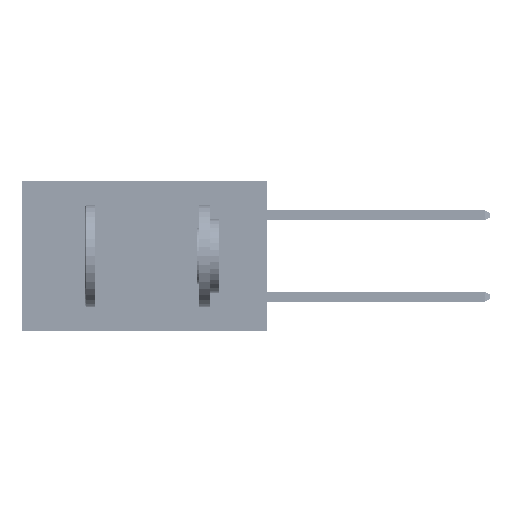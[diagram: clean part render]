
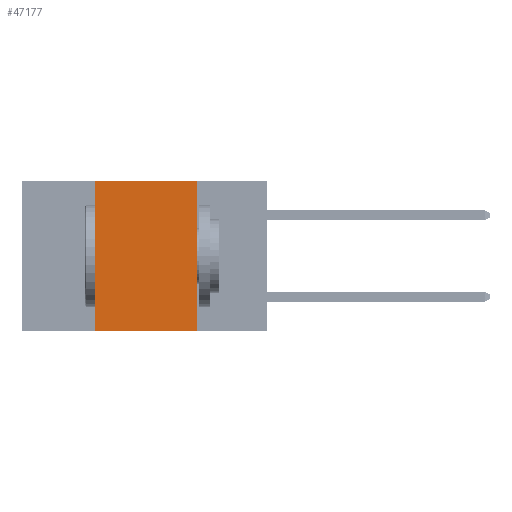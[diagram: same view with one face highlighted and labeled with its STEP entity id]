
A CAD part, left-side view. The second image highlights one B-rep face of the part: STEP entity #47177.
In plain terms, the highlighted planar face has unit normal (-1, 0, 0).
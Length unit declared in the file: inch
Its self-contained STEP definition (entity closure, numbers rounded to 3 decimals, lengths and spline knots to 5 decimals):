
#1394 = CARTESIAN_POINT ( 'NONE',  ( 0., 0.6, 0. ) ) ;
#2716 = DIRECTION ( 'NONE',  ( 0., -1., 0. ) ) ;
#3013 = EDGE_CURVE ( 'NONE', #48304, #9676, #44923, .T. ) ;
#9676 = VERTEX_POINT ( 'NONE', #44063 ) ;
#12251 = EDGE_CURVE ( 'NONE', #19786, #48304, #48145, .T. ) ;
#17034 = DIRECTION ( 'NONE',  ( 0., -1., 0. ) ) ;
#19220 = CARTESIAN_POINT ( 'NONE',  ( 0., 0.6, -0.37 ) ) ;
#19233 = CARTESIAN_POINT ( 'NONE',  ( 0., 0.42, 0. ) ) ;
#19470 = EDGE_CURVE ( 'NONE', #9676, #36220, #29450, .T. ) ;
#19753 = FACE_OUTER_BOUND ( 'NONE', #34911, .T. ) ;
#19786 = VERTEX_POINT ( 'NONE', #44908 ) ;
#21094 = VECTOR ( 'NONE', #17034, 39.37008 ) ;
#22067 = AXIS2_PLACEMENT_3D ( 'NONE', #28097, #32344, #24230 ) ;
#23722 = CARTESIAN_POINT ( 'NONE',  ( 0., 0.42, 0. ) ) ;
#24030 = ORIENTED_EDGE ( 'NONE', *, *, #12251, .F. ) ;
#24230 = DIRECTION ( 'NONE',  ( 0., 0., -1. ) ) ;
#24507 = ORIENTED_EDGE ( 'NONE', *, *, #19470, .F. ) ;
#27634 = ORIENTED_EDGE ( 'NONE', *, *, #33239, .T. ) ;
#28097 = CARTESIAN_POINT ( 'NONE',  ( 0., 0.6, 0. ) ) ;
#29450 = LINE ( 'NONE', #42570, #42639 ) ;
#30207 = VECTOR ( 'NONE', #2716, 39.37008 ) ;
#30304 = DIRECTION ( 'NONE',  ( 0., 0., -1. ) ) ;
#32344 = DIRECTION ( 'NONE',  ( 1., 0., 0. ) ) ;
#32692 = PLANE ( 'NONE',  #22067 ) ;
#33239 = EDGE_CURVE ( 'NONE', #19786, #36220, #43958, .T. ) ;
#34911 = EDGE_LOOP ( 'NONE', ( #24507, #38309, #24030, #27634 ) ) ;
#35054 = DIRECTION ( 'NONE',  ( 0., 0., 1. ) ) ;
#35658 = VECTOR ( 'NONE', #35054, 39.37008 ) ;
#36220 = VERTEX_POINT ( 'NONE', #47036 ) ;
#38309 = ORIENTED_EDGE ( 'NONE', *, *, #3013, .F. ) ;
#42570 = CARTESIAN_POINT ( 'NONE',  ( 0., 0.17, 0. ) ) ;
#42639 = VECTOR ( 'NONE', #30304, 39.37008 ) ;
#43958 = LINE ( 'NONE', #19220, #30207 ) ;
#44063 = CARTESIAN_POINT ( 'NONE',  ( 0., 0.17, 0. ) ) ;
#44908 = CARTESIAN_POINT ( 'NONE',  ( 0., 0.42, -0.37 ) ) ;
#44923 = LINE ( 'NONE', #1394, #21094 ) ;
#47036 = CARTESIAN_POINT ( 'NONE',  ( 0., 0.17, -0.37 ) ) ;
#47177 = ADVANCED_FACE ( 'NONE', ( #19753 ), #32692, .F. ) ;
#48145 = LINE ( 'NONE', #19233, #35658 ) ;
#48304 = VERTEX_POINT ( 'NONE', #23722 ) ;
